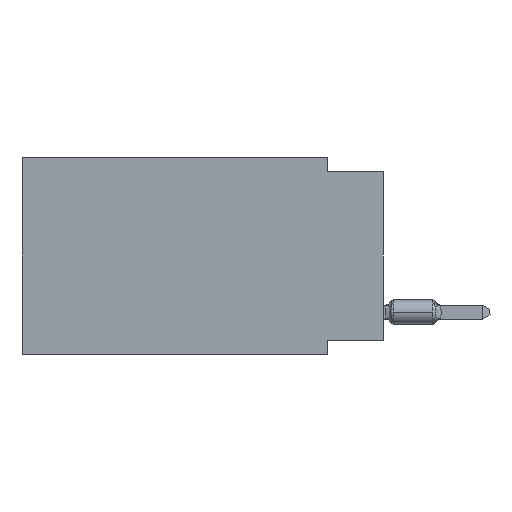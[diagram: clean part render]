
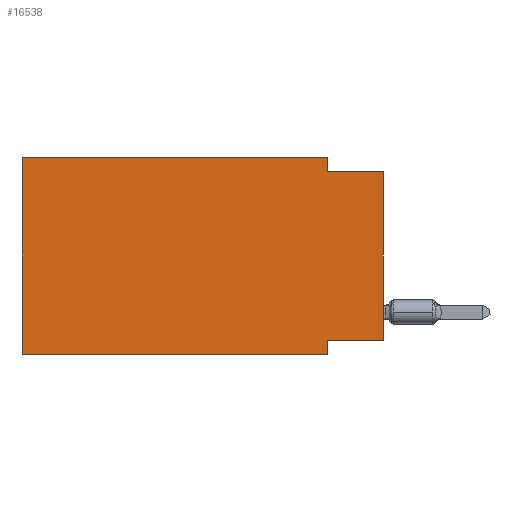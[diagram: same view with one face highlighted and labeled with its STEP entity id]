
A CAD part, left-side view. The second image highlights one B-rep face of the part: STEP entity #16538.
In plain terms, the highlighted planar face has unit normal (-1, 0, 0).
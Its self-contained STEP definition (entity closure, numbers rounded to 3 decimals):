
#351 = LINE ( 'NONE', #5106, #7777 ) ;
#364 = ORIENTED_EDGE ( 'NONE', *, *, #14557, .T. ) ;
#588 = LINE ( 'NONE', #21562, #16157 ) ;
#1075 = CARTESIAN_POINT ( 'NONE',  ( 0., 0., -0.635 ) ) ;
#1158 = VERTEX_POINT ( 'NONE', #11865 ) ;
#1384 = VERTEX_POINT ( 'NONE', #21443 ) ;
#1930 = VECTOR ( 'NONE', #5674, 1000. ) ;
#3348 = ORIENTED_EDGE ( 'NONE', *, *, #22113, .F. ) ;
#4055 = VECTOR ( 'NONE', #22119, 1000. ) ;
#4195 = CARTESIAN_POINT ( 'NONE',  ( 0., 16.383, 0. ) ) ;
#4583 = ORIENTED_EDGE ( 'NONE', *, *, #12813, .F. ) ;
#5106 = CARTESIAN_POINT ( 'NONE',  ( 0., 0., 0. ) ) ;
#5291 = DIRECTION ( 'NONE',  ( 0., 0., -1. ) ) ;
#5404 = DIRECTION ( 'NONE',  ( 1., 0., 0. ) ) ;
#5674 = DIRECTION ( 'NONE',  ( 0., 0., 1. ) ) ;
#5802 = EDGE_CURVE ( 'NONE', #16617, #7228, #588, .T. ) ;
#6090 = VERTEX_POINT ( 'NONE', #9039 ) ;
#6141 = DIRECTION ( 'NONE',  ( 0., 0., -1. ) ) ;
#6549 = ORIENTED_EDGE ( 'NONE', *, *, #5802, .F. ) ;
#7041 = AXIS2_PLACEMENT_3D ( 'NONE', #20934, #5404, #5291 ) ;
#7228 = VERTEX_POINT ( 'NONE', #18938 ) ;
#7310 = VECTOR ( 'NONE', #19162, 1000. ) ;
#7777 = VECTOR ( 'NONE', #17247, 1000. ) ;
#7943 = ORIENTED_EDGE ( 'NONE', *, *, #21596, .F. ) ;
#8903 = EDGE_CURVE ( 'NONE', #1158, #16617, #11516, .T. ) ;
#9039 = CARTESIAN_POINT ( 'NONE',  ( 0., 2.54, -8.89 ) ) ;
#9372 = CARTESIAN_POINT ( 'NONE',  ( 0., 0., -0.635 ) ) ;
#10502 = PLANE ( 'NONE',  #7041 ) ;
#11008 = VERTEX_POINT ( 'NONE', #9372 ) ;
#11286 = VECTOR ( 'NONE', #22148, 1000. ) ;
#11516 = LINE ( 'NONE', #20128, #14151 ) ;
#11865 = CARTESIAN_POINT ( 'NONE',  ( 0., 16.383, 0. ) ) ;
#12067 = ORIENTED_EDGE ( 'NONE', *, *, #8903, .F. ) ;
#12140 = LINE ( 'NONE', #20525, #7310 ) ;
#12731 = VERTEX_POINT ( 'NONE', #12980 ) ;
#12813 = EDGE_CURVE ( 'NONE', #1384, #1158, #16102, .T. ) ;
#12980 = CARTESIAN_POINT ( 'NONE',  ( 0., 2.54, -8.255 ) ) ;
#13078 = EDGE_CURVE ( 'NONE', #12731, #6090, #22234, .T. ) ;
#13312 = ORIENTED_EDGE ( 'NONE', *, *, #13078, .F. ) ;
#13458 = FACE_OUTER_BOUND ( 'NONE', #13959, .T. ) ;
#13830 = CARTESIAN_POINT ( 'NONE',  ( 0., 0., -8.255 ) ) ;
#13959 = EDGE_LOOP ( 'NONE', ( #364, #7943, #6549, #12067, #4583, #17421, #13312, #3348 ) ) ;
#14151 = VECTOR ( 'NONE', #21723, 1000. ) ;
#14557 = EDGE_CURVE ( 'NONE', #22094, #11008, #351, .T. ) ;
#15349 = LINE ( 'NONE', #1075, #11286 ) ;
#16102 = LINE ( 'NONE', #4195, #1930 ) ;
#16157 = VECTOR ( 'NONE', #6141, 1000. ) ;
#16538 = ADVANCED_FACE ( 'NONE', ( #13458 ), #10502, .F. ) ;
#16617 = VERTEX_POINT ( 'NONE', #17314 ) ;
#17247 = DIRECTION ( 'NONE',  ( 0., 0., 1. ) ) ;
#17314 = CARTESIAN_POINT ( 'NONE',  ( 0., 2.54, 0. ) ) ;
#17421 = ORIENTED_EDGE ( 'NONE', *, *, #20322, .T. ) ;
#17677 = LINE ( 'NONE', #19482, #21811 ) ;
#18938 = CARTESIAN_POINT ( 'NONE',  ( 0., 2.54, -0.635 ) ) ;
#19151 = DIRECTION ( 'NONE',  ( 0., -1., 0. ) ) ;
#19162 = DIRECTION ( 'NONE',  ( 0., 1., 0. ) ) ;
#19482 = CARTESIAN_POINT ( 'NONE',  ( 0., 16.383, -8.89 ) ) ;
#20128 = CARTESIAN_POINT ( 'NONE',  ( 0., 16.383, 0. ) ) ;
#20322 = EDGE_CURVE ( 'NONE', #1384, #6090, #17677, .T. ) ;
#20525 = CARTESIAN_POINT ( 'NONE',  ( 0., 0., -8.255 ) ) ;
#20934 = CARTESIAN_POINT ( 'NONE',  ( 0., 16.383, 0. ) ) ;
#21443 = CARTESIAN_POINT ( 'NONE',  ( 0., 16.383, -8.89 ) ) ;
#21562 = CARTESIAN_POINT ( 'NONE',  ( 0., 2.54, 0. ) ) ;
#21596 = EDGE_CURVE ( 'NONE', #7228, #11008, #15349, .T. ) ;
#21723 = DIRECTION ( 'NONE',  ( 0., -1., 0. ) ) ;
#21811 = VECTOR ( 'NONE', #19151, 1000. ) ;
#21895 = CARTESIAN_POINT ( 'NONE',  ( 0., 2.54, -8.89 ) ) ;
#22094 = VERTEX_POINT ( 'NONE', #13830 ) ;
#22113 = EDGE_CURVE ( 'NONE', #22094, #12731, #12140, .T. ) ;
#22119 = DIRECTION ( 'NONE',  ( 0., 0., -1. ) ) ;
#22148 = DIRECTION ( 'NONE',  ( 0., -1., 0. ) ) ;
#22234 = LINE ( 'NONE', #21895, #4055 ) ;
